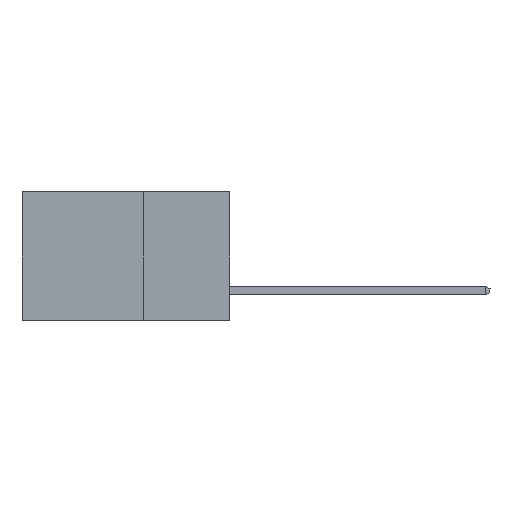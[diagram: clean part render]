
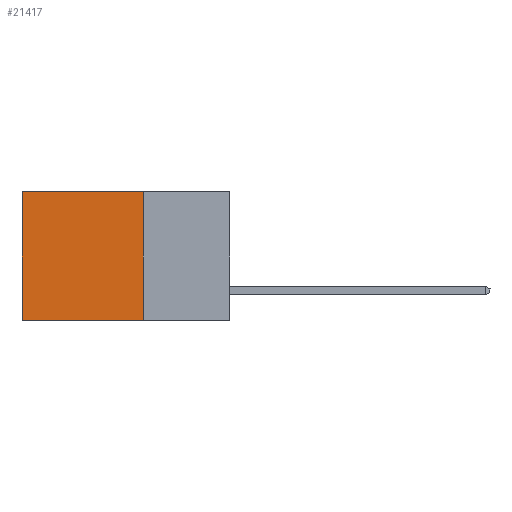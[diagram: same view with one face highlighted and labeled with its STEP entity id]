
A CAD part, left-side view. The second image highlights one B-rep face of the part: STEP entity #21417.
In plain terms, the highlighted planar face has unit normal (-1, 0, 0).
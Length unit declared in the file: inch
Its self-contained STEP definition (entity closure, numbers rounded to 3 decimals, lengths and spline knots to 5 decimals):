
#282 = VECTOR ( 'NONE', #702, 39.37008 ) ;
#402 = LINE ( 'NONE', #13528, #6053 ) ;
#499 = DIRECTION ( 'NONE',  ( 1., 0., 0. ) ) ;
#702 = DIRECTION ( 'NONE',  ( 0., 1., 0. ) ) ;
#980 = EDGE_CURVE ( 'NONE', #13545, #11616, #2069, .T. ) ;
#2069 = LINE ( 'NONE', #15188, #282 ) ;
#3033 = LINE ( 'NONE', #6365, #7426 ) ;
#3596 = VECTOR ( 'NONE', #9018, 39.37008 ) ;
#4543 = CARTESIAN_POINT ( 'NONE',  ( 0.2615, 0.6, -0.37 ) ) ;
#5347 = CARTESIAN_POINT ( 'NONE',  ( 0.2615, 0.6, 0. ) ) ;
#6053 = VECTOR ( 'NONE', #16728, 39.37008 ) ;
#6365 = CARTESIAN_POINT ( 'NONE',  ( 0.2615, 0.6, -0.37 ) ) ;
#7232 = VERTEX_POINT ( 'NONE', #5347 ) ;
#7426 = VECTOR ( 'NONE', #10503, 39.37008 ) ;
#7879 = ORIENTED_EDGE ( 'NONE', *, *, #980, .F. ) ;
#8457 = DIRECTION ( 'NONE',  ( 0., 0., -1. ) ) ;
#8969 = AXIS2_PLACEMENT_3D ( 'NONE', #13732, #499, #8457 ) ;
#9018 = DIRECTION ( 'NONE',  ( 0., 0., -1. ) ) ;
#10134 = ORIENTED_EDGE ( 'NONE', *, *, #10861, .T. ) ;
#10503 = DIRECTION ( 'NONE',  ( 0., 0., -1. ) ) ;
#10861 = EDGE_CURVE ( 'NONE', #23565, #7232, #402, .T. ) ;
#11616 = VERTEX_POINT ( 'NONE', #4543 ) ;
#11906 = ORIENTED_EDGE ( 'NONE', *, *, #14005, .T. ) ;
#12471 = CARTESIAN_POINT ( 'NONE',  ( 0.2615, 0.25, 0. ) ) ;
#12569 = CARTESIAN_POINT ( 'NONE',  ( 0.2615, 0.25, -0.37 ) ) ;
#13528 = CARTESIAN_POINT ( 'NONE',  ( 0.2615, 0.25, 0. ) ) ;
#13545 = VERTEX_POINT ( 'NONE', #14352 ) ;
#13612 = FACE_OUTER_BOUND ( 'NONE', #23314, .T. ) ;
#13732 = CARTESIAN_POINT ( 'NONE',  ( 0.2615, 0.25, -0.37 ) ) ;
#14005 = EDGE_CURVE ( 'NONE', #7232, #11616, #3033, .T. ) ;
#14352 = CARTESIAN_POINT ( 'NONE',  ( 0.2615, 0.25, -0.37 ) ) ;
#15157 = ORIENTED_EDGE ( 'NONE', *, *, #18679, .F. ) ;
#15188 = CARTESIAN_POINT ( 'NONE',  ( 0.2615, 0.25, -0.37 ) ) ;
#16728 = DIRECTION ( 'NONE',  ( 0., 1., 0. ) ) ;
#18679 = EDGE_CURVE ( 'NONE', #23565, #13545, #22033, .T. ) ;
#21417 = ADVANCED_FACE ( 'NONE', ( #13612 ), #23071, .F. ) ;
#22033 = LINE ( 'NONE', #12569, #3596 ) ;
#23071 = PLANE ( 'NONE',  #8969 ) ;
#23314 = EDGE_LOOP ( 'NONE', ( #11906, #7879, #15157, #10134 ) ) ;
#23565 = VERTEX_POINT ( 'NONE', #12471 ) ;
